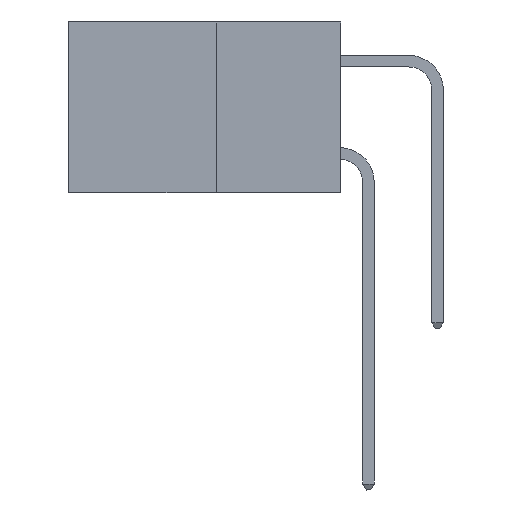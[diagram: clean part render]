
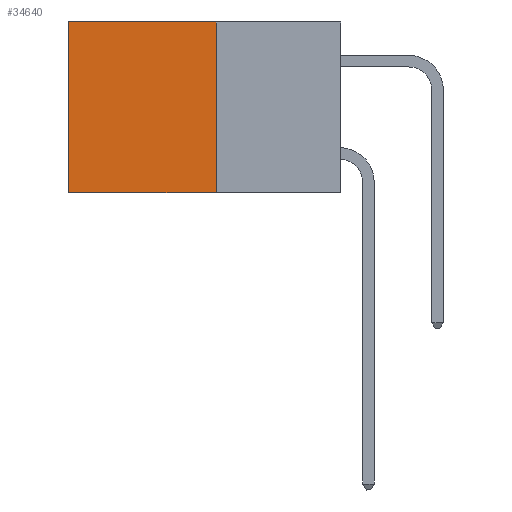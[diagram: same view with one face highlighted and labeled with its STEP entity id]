
A CAD part, left-side view. The second image highlights one B-rep face of the part: STEP entity #34640.
In plain terms, the highlighted planar face has unit normal (-1, 0, 0).
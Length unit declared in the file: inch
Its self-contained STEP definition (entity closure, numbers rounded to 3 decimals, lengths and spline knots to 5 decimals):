
#615 = EDGE_CURVE ( 'NONE', #33380, #29782, #21295, .T. ) ;
#634 = VECTOR ( 'NONE', #9346, 39.37008 ) ;
#731 = VERTEX_POINT ( 'NONE', #27374 ) ;
#5919 = VECTOR ( 'NONE', #9247, 39.37008 ) ;
#6203 = CARTESIAN_POINT ( 'NONE',  ( 0.277, 0.27, -0.37 ) ) ;
#7405 = ORIENTED_EDGE ( 'NONE', *, *, #24619, .T. ) ;
#8526 = VECTOR ( 'NONE', #16629, 39.37008 ) ;
#8553 = LINE ( 'NONE', #11977, #5919 ) ;
#8864 = ORIENTED_EDGE ( 'NONE', *, *, #615, .F. ) ;
#8912 = DIRECTION ( 'NONE',  ( 1., 0., 0. ) ) ;
#9035 = PLANE ( 'NONE',  #19205 ) ;
#9247 = DIRECTION ( 'NONE',  ( 0., 0., -1. ) ) ;
#9346 = DIRECTION ( 'NONE',  ( 0., 1., 0. ) ) ;
#9411 = LINE ( 'NONE', #30275, #8526 ) ;
#9842 = CARTESIAN_POINT ( 'NONE',  ( 0.277, 0.27, 0. ) ) ;
#11891 = DIRECTION ( 'NONE',  ( 0., 0., -1. ) ) ;
#11977 = CARTESIAN_POINT ( 'NONE',  ( 0.277, 0.27, -0.37 ) ) ;
#16069 = LINE ( 'NONE', #9842, #22535 ) ;
#16629 = DIRECTION ( 'NONE',  ( 0., 0., -1. ) ) ;
#19205 = AXIS2_PLACEMENT_3D ( 'NONE', #6203, #8912, #11891 ) ;
#21295 = LINE ( 'NONE', #31542, #634 ) ;
#22121 = VERTEX_POINT ( 'NONE', #31312 ) ;
#22535 = VECTOR ( 'NONE', #26419, 39.37008 ) ;
#22757 = CARTESIAN_POINT ( 'NONE',  ( 0.277, 0.27, -0.37 ) ) ;
#23781 = EDGE_LOOP ( 'NONE', ( #29218, #8864, #30206, #7405 ) ) ;
#24619 = EDGE_CURVE ( 'NONE', #731, #22121, #16069, .T. ) ;
#24693 = CARTESIAN_POINT ( 'NONE',  ( 0.277, 0.59, -0.37 ) ) ;
#26419 = DIRECTION ( 'NONE',  ( 0., 1., 0. ) ) ;
#27374 = CARTESIAN_POINT ( 'NONE',  ( 0.277, 0.27, 0. ) ) ;
#29218 = ORIENTED_EDGE ( 'NONE', *, *, #29795, .T. ) ;
#29782 = VERTEX_POINT ( 'NONE', #24693 ) ;
#29795 = EDGE_CURVE ( 'NONE', #22121, #29782, #9411, .T. ) ;
#30206 = ORIENTED_EDGE ( 'NONE', *, *, #33476, .F. ) ;
#30275 = CARTESIAN_POINT ( 'NONE',  ( 0.277, 0.59, -0.37 ) ) ;
#31312 = CARTESIAN_POINT ( 'NONE',  ( 0.277, 0.59, 0. ) ) ;
#31542 = CARTESIAN_POINT ( 'NONE',  ( 0.277, 0.27, -0.37 ) ) ;
#33380 = VERTEX_POINT ( 'NONE', #22757 ) ;
#33476 = EDGE_CURVE ( 'NONE', #731, #33380, #8553, .T. ) ;
#33919 = FACE_OUTER_BOUND ( 'NONE', #23781, .T. ) ;
#34640 = ADVANCED_FACE ( 'NONE', ( #33919 ), #9035, .F. ) ;
